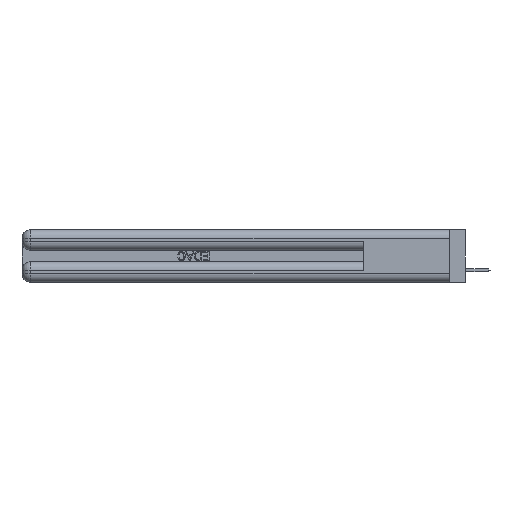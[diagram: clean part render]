
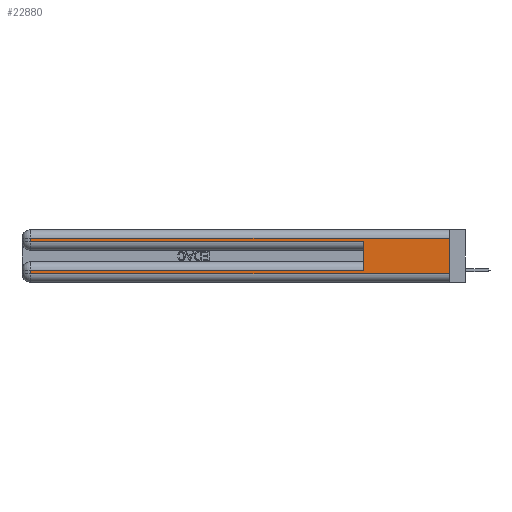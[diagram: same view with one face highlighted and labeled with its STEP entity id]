
A CAD part, left-side view. The second image highlights one B-rep face of the part: STEP entity #22880.
In plain terms, the highlighted planar face has unit normal (-1, 0, 0).
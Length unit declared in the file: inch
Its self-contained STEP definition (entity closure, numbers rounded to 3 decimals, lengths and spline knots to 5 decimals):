
#78 = FACE_OUTER_BOUND ( 'NONE', #34945, .T. ) ;
#87 = LINE ( 'NONE', #13837, #554 ) ;
#531 = CARTESIAN_POINT ( 'NONE',  ( 0., 0., 0.37 ) ) ;
#554 = VECTOR ( 'NONE', #21524, 39.37008 ) ;
#1721 = EDGE_CURVE ( 'NONE', #28126, #14985, #15235, .T. ) ;
#1842 = CARTESIAN_POINT ( 'NONE',  ( 0., 0., 0.31 ) ) ;
#3678 = CARTESIAN_POINT ( 'NONE',  ( 0., 0., 0.06 ) ) ;
#5793 = VERTEX_POINT ( 'NONE', #18169 ) ;
#5922 = ORIENTED_EDGE ( 'NONE', *, *, #32256, .T. ) ;
#6670 = CARTESIAN_POINT ( 'NONE',  ( 0., 2.94, 0.37 ) ) ;
#6961 = LINE ( 'NONE', #45606, #14741 ) ;
#7229 = ORIENTED_EDGE ( 'NONE', *, *, #1721, .F. ) ;
#7849 = DIRECTION ( 'NONE',  ( 0., -1., 0. ) ) ;
#9578 = DIRECTION ( 'NONE',  ( 0., 1., 0. ) ) ;
#9741 = CARTESIAN_POINT ( 'NONE',  ( 0., 0.6, 0.085 ) ) ;
#9953 = ORIENTED_EDGE ( 'NONE', *, *, #42368, .T. ) ;
#10035 = VECTOR ( 'NONE', #27265, 39.37008 ) ;
#12355 = DIRECTION ( 'NONE',  ( 0., 0., -1. ) ) ;
#12618 = LINE ( 'NONE', #6670, #40052 ) ;
#13611 = CARTESIAN_POINT ( 'NONE',  ( 0., 2.94, 0.285 ) ) ;
#13638 = LINE ( 'NONE', #18829, #10035 ) ;
#13837 = CARTESIAN_POINT ( 'NONE',  ( 0., 2.94, 0.37 ) ) ;
#14741 = VECTOR ( 'NONE', #7849, 39.37008 ) ;
#14985 = VERTEX_POINT ( 'NONE', #44165 ) ;
#15235 = LINE ( 'NONE', #21815, #40284 ) ;
#15350 = CARTESIAN_POINT ( 'NONE',  ( 0., 2.94, 0.085 ) ) ;
#15426 = AXIS2_PLACEMENT_3D ( 'NONE', #43208, #24217, #12355 ) ;
#17651 = VERTEX_POINT ( 'NONE', #13611 ) ;
#17982 = ORIENTED_EDGE ( 'NONE', *, *, #24655, .F. ) ;
#18169 = CARTESIAN_POINT ( 'NONE',  ( 0., 2.94, 0.31 ) ) ;
#18829 = CARTESIAN_POINT ( 'NONE',  ( 0., 0., 0.31 ) ) ;
#18906 = VERTEX_POINT ( 'NONE', #1842 ) ;
#19602 = LINE ( 'NONE', #28595, #26803 ) ;
#21524 = DIRECTION ( 'NONE',  ( 0., 0., -1. ) ) ;
#21815 = CARTESIAN_POINT ( 'NONE',  ( 0., 0.6, 0.145 ) ) ;
#22120 = EDGE_CURVE ( 'NONE', #17651, #14985, #27518, .T. ) ;
#22145 = DIRECTION ( 'NONE',  ( 0., 0., 1. ) ) ;
#22270 = ORIENTED_EDGE ( 'NONE', *, *, #22120, .T. ) ;
#22880 = ADVANCED_FACE ( 'NONE', ( #78 ), #24039, .F. ) ;
#23295 = ORIENTED_EDGE ( 'NONE', *, *, #28025, .T. ) ;
#24039 = PLANE ( 'NONE',  #15426 ) ;
#24217 = DIRECTION ( 'NONE',  ( 1., 0., 0. ) ) ;
#24300 = LINE ( 'NONE', #531, #47567 ) ;
#24655 = EDGE_CURVE ( 'NONE', #18906, #25021, #24300, .T. ) ;
#25021 = VERTEX_POINT ( 'NONE', #3678 ) ;
#25357 = EDGE_CURVE ( 'NONE', #30621, #25021, #6961, .T. ) ;
#25741 = CARTESIAN_POINT ( 'NONE',  ( 0., 2.94, 0.06 ) ) ;
#26803 = VECTOR ( 'NONE', #9578, 39.37008 ) ;
#27265 = DIRECTION ( 'NONE',  ( 0., 1., 0. ) ) ;
#27518 = LINE ( 'NONE', #28773, #35955 ) ;
#28025 = EDGE_CURVE ( 'NONE', #28126, #28941, #19602, .T. ) ;
#28069 = ORIENTED_EDGE ( 'NONE', *, *, #25357, .T. ) ;
#28126 = VERTEX_POINT ( 'NONE', #9741 ) ;
#28595 = CARTESIAN_POINT ( 'NONE',  ( 0., 0., 0.085 ) ) ;
#28773 = CARTESIAN_POINT ( 'NONE',  ( 0., 0., 0.285 ) ) ;
#28941 = VERTEX_POINT ( 'NONE', #15350 ) ;
#30621 = VERTEX_POINT ( 'NONE', #25741 ) ;
#32256 = EDGE_CURVE ( 'NONE', #5793, #17651, #12618, .T. ) ;
#34945 = EDGE_LOOP ( 'NONE', ( #17982, #9953, #5922, #22270, #7229, #23295, #35788, #28069 ) ) ;
#35612 = DIRECTION ( 'NONE',  ( 0., 0., -1. ) ) ;
#35788 = ORIENTED_EDGE ( 'NONE', *, *, #47817, .T. ) ;
#35955 = VECTOR ( 'NONE', #44302, 39.37008 ) ;
#40052 = VECTOR ( 'NONE', #45067, 39.37008 ) ;
#40284 = VECTOR ( 'NONE', #22145, 39.37008 ) ;
#42368 = EDGE_CURVE ( 'NONE', #18906, #5793, #13638, .T. ) ;
#43208 = CARTESIAN_POINT ( 'NONE',  ( 0., 0., 0.37 ) ) ;
#44165 = CARTESIAN_POINT ( 'NONE',  ( 0., 0.6, 0.285 ) ) ;
#44302 = DIRECTION ( 'NONE',  ( 0., -1., 0. ) ) ;
#45067 = DIRECTION ( 'NONE',  ( 0., 0., -1. ) ) ;
#45606 = CARTESIAN_POINT ( 'NONE',  ( 0., 0., 0.06 ) ) ;
#47567 = VECTOR ( 'NONE', #35612, 39.37008 ) ;
#47817 = EDGE_CURVE ( 'NONE', #28941, #30621, #87, .T. ) ;
